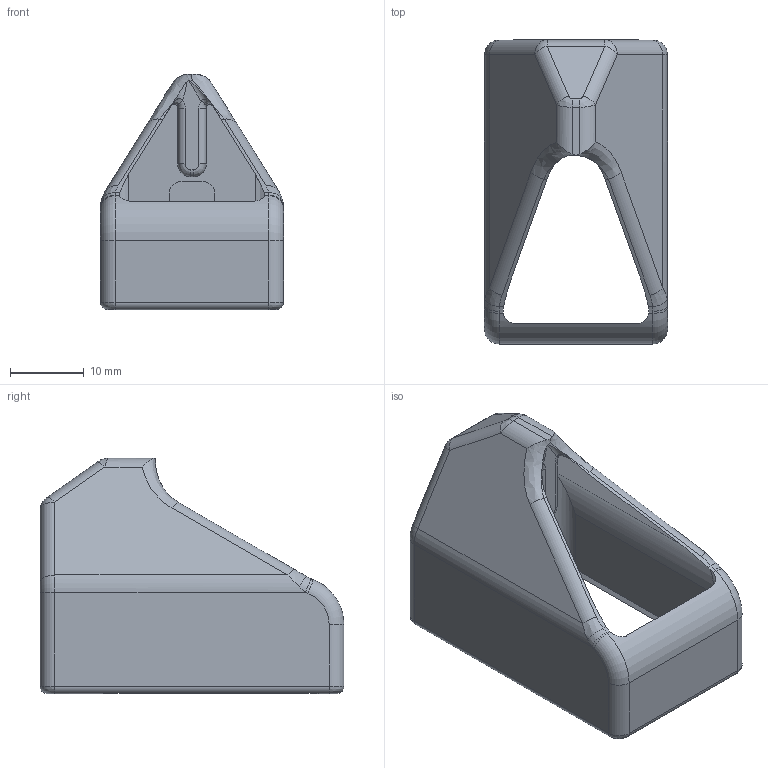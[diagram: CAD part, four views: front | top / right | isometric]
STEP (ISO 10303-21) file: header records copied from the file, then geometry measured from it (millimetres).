
FILE_DESCRIPTION(/* description */ (''),/* implementation_level */ '2;1');
FILE_NAME(/* name */ 'VZ 61 .22 LR Speed Loader v5.step',/* time_stamp */ '2021-02-13T01:06:18-05:00',/* author */ (''),/* organization */ (''),/* preprocessor_version */ 'ST-DEVELOPER v18.1',/* originating_system */ 'Autodesk Translation Framework v9.7.1.1290',/* authorisation */ '');
FILE_SCHEMA (('AUTOMOTIVE_DESIGN { 1 0 10303 214 3 1 1 }'));
Length unit declared in the file: millimetre
Products named in the file (2): VZ 61 .22 LR Speed Loader; VZ61 22LR Speedloader Body
Assembly tree (1 placements, depth 2):
  VZ 61 .22 LR Speed Loader
    VZ61 22LR Speedloader Body
Bounding box: 24.82 x 41.2 x 31.9 mm (x, y, z)
Volume: 7945.4 mm3; surface area: 5889.2 mm2
Topology: 1 solids, 1 shells, 123 faces, 308 edges, 183 vertices
Faces by surface type: cylinder 48, plane 35, bspline 22, torus 12, cone 4, sphere 2
Entity records: 4224 total; most frequent: CARTESIAN_POINT 1305, ORIENTED_EDGE 612, DIRECTION 607, EDGE_CURVE 306, AXIS2_PLACEMENT_3D 235, VERTEX_POINT 183, LINE 137, VECTOR 137
